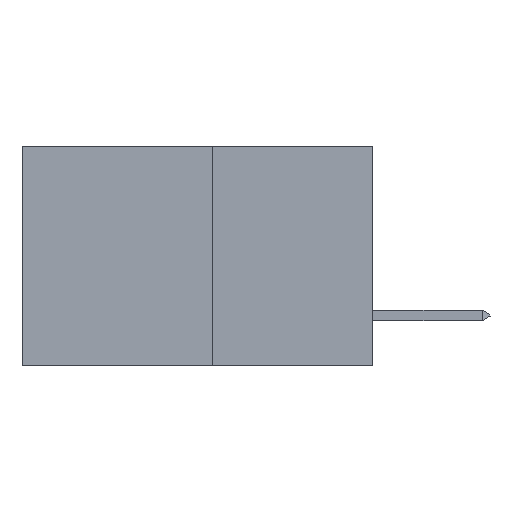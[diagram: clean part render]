
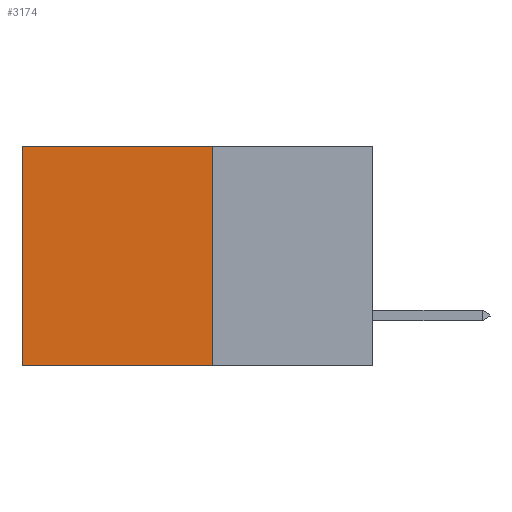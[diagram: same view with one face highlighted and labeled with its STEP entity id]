
A CAD part, left-side view. The second image highlights one B-rep face of the part: STEP entity #3174.
In plain terms, the highlighted planar face has unit normal (-1, 0, 0).
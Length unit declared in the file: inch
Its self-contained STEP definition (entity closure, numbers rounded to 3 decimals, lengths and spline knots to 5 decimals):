
#428 = EDGE_LOOP ( 'NONE', ( #5060, #7252, #13562, #814 ) ) ;
#814 = ORIENTED_EDGE ( 'NONE', *, *, #1561, .T. ) ;
#1224 = EDGE_CURVE ( 'NONE', #10958, #16242, #10168, .T. ) ;
#1561 = EDGE_CURVE ( 'NONE', #6393, #10958, #3999, .T. ) ;
#1911 = LINE ( 'NONE', #11526, #14993 ) ;
#2090 = CARTESIAN_POINT ( 'NONE',  ( 0.277, 0.27, -0.37 ) ) ;
#2329 = VERTEX_POINT ( 'NONE', #2090 ) ;
#2743 = DIRECTION ( 'NONE',  ( 1., 0., 0. ) ) ;
#3079 = CARTESIAN_POINT ( 'NONE',  ( 0.277, 0.59, 0. ) ) ;
#3174 = ADVANCED_FACE ( 'NONE', ( #15046 ), #7753, .F. ) ;
#3427 = VECTOR ( 'NONE', #11647, 39.37008 ) ;
#3999 = LINE ( 'NONE', #15896, #13686 ) ;
#4903 = CARTESIAN_POINT ( 'NONE',  ( 0.277, 0.27, -0.37 ) ) ;
#5060 = ORIENTED_EDGE ( 'NONE', *, *, #1224, .T. ) ;
#5654 = DIRECTION ( 'NONE',  ( 0., 1., 0. ) ) ;
#6393 = VERTEX_POINT ( 'NONE', #11286 ) ;
#7252 = ORIENTED_EDGE ( 'NONE', *, *, #9556, .F. ) ;
#7753 = PLANE ( 'NONE',  #9936 ) ;
#7804 = DIRECTION ( 'NONE',  ( 0., 0., -1. ) ) ;
#9556 = EDGE_CURVE ( 'NONE', #2329, #16242, #10916, .T. ) ;
#9936 = AXIS2_PLACEMENT_3D ( 'NONE', #15357, #2743, #11579 ) ;
#10168 = LINE ( 'NONE', #12222, #3427 ) ;
#10529 = VECTOR ( 'NONE', #11189, 39.37008 ) ;
#10916 = LINE ( 'NONE', #4903, #10529 ) ;
#10958 = VERTEX_POINT ( 'NONE', #3079 ) ;
#11189 = DIRECTION ( 'NONE',  ( 0., 1., 0. ) ) ;
#11286 = CARTESIAN_POINT ( 'NONE',  ( 0.277, 0.27, 0. ) ) ;
#11526 = CARTESIAN_POINT ( 'NONE',  ( 0.277, 0.27, -0.37 ) ) ;
#11579 = DIRECTION ( 'NONE',  ( 0., 0., -1. ) ) ;
#11647 = DIRECTION ( 'NONE',  ( 0., 0., -1. ) ) ;
#12222 = CARTESIAN_POINT ( 'NONE',  ( 0.277, 0.59, -0.37 ) ) ;
#12640 = CARTESIAN_POINT ( 'NONE',  ( 0.277, 0.59, -0.37 ) ) ;
#13107 = EDGE_CURVE ( 'NONE', #6393, #2329, #1911, .T. ) ;
#13562 = ORIENTED_EDGE ( 'NONE', *, *, #13107, .F. ) ;
#13686 = VECTOR ( 'NONE', #5654, 39.37008 ) ;
#14993 = VECTOR ( 'NONE', #7804, 39.37008 ) ;
#15046 = FACE_OUTER_BOUND ( 'NONE', #428, .T. ) ;
#15357 = CARTESIAN_POINT ( 'NONE',  ( 0.277, 0.27, -0.37 ) ) ;
#15896 = CARTESIAN_POINT ( 'NONE',  ( 0.277, 0.27, 0. ) ) ;
#16242 = VERTEX_POINT ( 'NONE', #12640 ) ;
